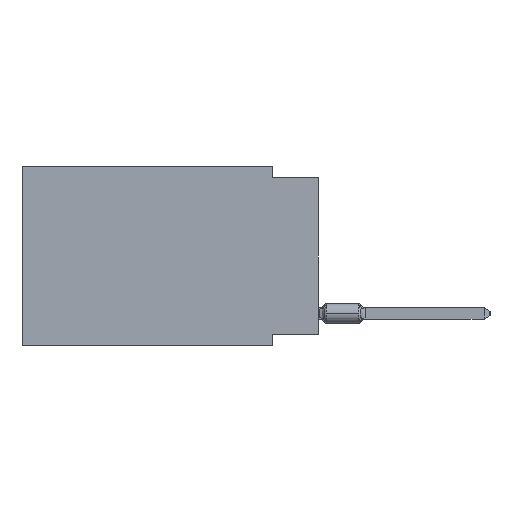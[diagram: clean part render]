
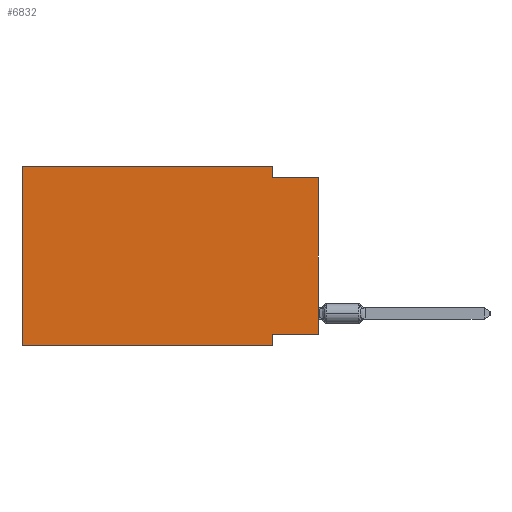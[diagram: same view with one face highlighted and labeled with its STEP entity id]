
A CAD part, left-side view. The second image highlights one B-rep face of the part: STEP entity #6832.
In plain terms, the highlighted planar face has unit normal (-1, 0, 0).
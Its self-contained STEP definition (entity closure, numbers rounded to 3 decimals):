
#485 = CARTESIAN_POINT ( 'NONE',  ( 0., 16.383, 0. ) ) ;
#3169 = LINE ( 'NONE', #52072, #79300 ) ;
#4884 = DIRECTION ( 'NONE',  ( 0., 0., 1. ) ) ;
#5029 = LINE ( 'NONE', #74860, #25971 ) ;
#5280 = LINE ( 'NONE', #10665, #48462 ) ;
#6832 = ADVANCED_FACE ( 'NONE', ( #55070 ), #48898, .F. ) ;
#6840 = LINE ( 'NONE', #32287, #29456 ) ;
#10013 = CARTESIAN_POINT ( 'NONE',  ( 0., 2.54, 0. ) ) ;
#10401 = CARTESIAN_POINT ( 'NONE',  ( 0., 2.54, -0.635 ) ) ;
#10665 = CARTESIAN_POINT ( 'NONE',  ( 0., 16.383, 0. ) ) ;
#11412 = DIRECTION ( 'NONE',  ( 0., 0., 1. ) ) ;
#12375 = AXIS2_PLACEMENT_3D ( 'NONE', #18911, #31643, #43970 ) ;
#13848 = VERTEX_POINT ( 'NONE', #485 ) ;
#14590 = ORIENTED_EDGE ( 'NONE', *, *, #32305, .F. ) ;
#16951 = DIRECTION ( 'NONE',  ( 0., 0., -1. ) ) ;
#18911 = CARTESIAN_POINT ( 'NONE',  ( 0., 16.383, 0. ) ) ;
#19571 = CARTESIAN_POINT ( 'NONE',  ( 0., 0., 0. ) ) ;
#21999 = ORIENTED_EDGE ( 'NONE', *, *, #73201, .F. ) ;
#22328 = ORIENTED_EDGE ( 'NONE', *, *, #77025, .F. ) ;
#25971 = VECTOR ( 'NONE', #16951, 1000. ) ;
#25998 = EDGE_CURVE ( 'NONE', #32578, #42884, #50784, .T. ) ;
#26596 = VERTEX_POINT ( 'NONE', #10013 ) ;
#27831 = DIRECTION ( 'NONE',  ( 0., -1., 0. ) ) ;
#28562 = LINE ( 'NONE', #60589, #59416 ) ;
#29456 = VECTOR ( 'NONE', #51552, 1000. ) ;
#29633 = LINE ( 'NONE', #68217, #52707 ) ;
#29818 = CARTESIAN_POINT ( 'NONE',  ( 0., 0., -0.635 ) ) ;
#30586 = EDGE_CURVE ( 'NONE', #35585, #13848, #5280, .T. ) ;
#31625 = ORIENTED_EDGE ( 'NONE', *, *, #30586, .F. ) ;
#31643 = DIRECTION ( 'NONE',  ( 1., 0., 0. ) ) ;
#32287 = CARTESIAN_POINT ( 'NONE',  ( 0., 16.383, 0. ) ) ;
#32305 = EDGE_CURVE ( 'NONE', #13848, #26596, #6840, .T. ) ;
#32578 = VERTEX_POINT ( 'NONE', #51809 ) ;
#34320 = CARTESIAN_POINT ( 'NONE',  ( 0., 2.54, -9.906 ) ) ;
#35585 = VERTEX_POINT ( 'NONE', #49488 ) ;
#36092 = ORIENTED_EDGE ( 'NONE', *, *, #51390, .F. ) ;
#38762 = VECTOR ( 'NONE', #59791, 1000. ) ;
#40333 = EDGE_LOOP ( 'NONE', ( #76445, #22328, #36092, #14590, #31625, #78793, #66360, #21999 ) ) ;
#42884 = VERTEX_POINT ( 'NONE', #29818 ) ;
#43970 = DIRECTION ( 'NONE',  ( 0., 0., -1. ) ) ;
#47757 = VERTEX_POINT ( 'NONE', #73837 ) ;
#48088 = EDGE_CURVE ( 'NONE', #50295, #47757, #72944, .T. ) ;
#48462 = VECTOR ( 'NONE', #4884, 1000. ) ;
#48898 = PLANE ( 'NONE',  #12375 ) ;
#49488 = CARTESIAN_POINT ( 'NONE',  ( 0., 16.383, -9.906 ) ) ;
#50295 = VERTEX_POINT ( 'NONE', #70183 ) ;
#50784 = LINE ( 'NONE', #19571, #56949 ) ;
#51390 = EDGE_CURVE ( 'NONE', #26596, #59805, #5029, .T. ) ;
#51552 = DIRECTION ( 'NONE',  ( 0., -1., 0. ) ) ;
#51809 = CARTESIAN_POINT ( 'NONE',  ( 0., 0., -9.271 ) ) ;
#52072 = CARTESIAN_POINT ( 'NONE',  ( 0., 16.383, -9.906 ) ) ;
#52707 = VECTOR ( 'NONE', #80568, 1000. ) ;
#55070 = FACE_OUTER_BOUND ( 'NONE', #40333, .T. ) ;
#56949 = VECTOR ( 'NONE', #11412, 1000. ) ;
#58279 = EDGE_CURVE ( 'NONE', #35585, #47757, #3169, .T. ) ;
#59416 = VECTOR ( 'NONE', #59780, 1000. ) ;
#59780 = DIRECTION ( 'NONE',  ( 0., 1., 0. ) ) ;
#59791 = DIRECTION ( 'NONE',  ( 0., 0., -1. ) ) ;
#59805 = VERTEX_POINT ( 'NONE', #10401 ) ;
#60589 = CARTESIAN_POINT ( 'NONE',  ( 0., 0., -9.271 ) ) ;
#66360 = ORIENTED_EDGE ( 'NONE', *, *, #48088, .F. ) ;
#68217 = CARTESIAN_POINT ( 'NONE',  ( 0., 0., -0.635 ) ) ;
#70183 = CARTESIAN_POINT ( 'NONE',  ( 0., 2.54, -9.271 ) ) ;
#72944 = LINE ( 'NONE', #34320, #38762 ) ;
#73201 = EDGE_CURVE ( 'NONE', #32578, #50295, #28562, .T. ) ;
#73837 = CARTESIAN_POINT ( 'NONE',  ( 0., 2.54, -9.906 ) ) ;
#74860 = CARTESIAN_POINT ( 'NONE',  ( 0., 2.54, 0. ) ) ;
#76445 = ORIENTED_EDGE ( 'NONE', *, *, #25998, .T. ) ;
#77025 = EDGE_CURVE ( 'NONE', #59805, #42884, #29633, .T. ) ;
#78793 = ORIENTED_EDGE ( 'NONE', *, *, #58279, .T. ) ;
#79300 = VECTOR ( 'NONE', #27831, 1000. ) ;
#80568 = DIRECTION ( 'NONE',  ( 0., -1., 0. ) ) ;
